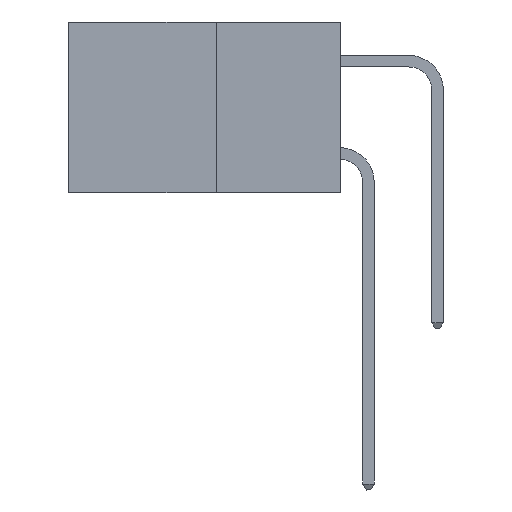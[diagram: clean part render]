
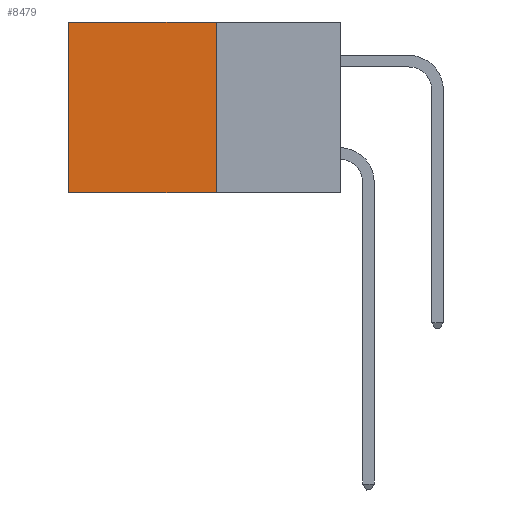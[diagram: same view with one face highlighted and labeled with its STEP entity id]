
A CAD part, left-side view. The second image highlights one B-rep face of the part: STEP entity #8479.
In plain terms, the highlighted planar face has unit normal (-1, 0, 0).
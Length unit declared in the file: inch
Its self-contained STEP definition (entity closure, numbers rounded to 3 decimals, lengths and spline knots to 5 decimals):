
#116 = VERTEX_POINT ( 'NONE', #1490 ) ;
#1490 = CARTESIAN_POINT ( 'NONE',  ( 0.277, 0.59, -0.37 ) ) ;
#2420 = VERTEX_POINT ( 'NONE', #4326 ) ;
#3546 = VERTEX_POINT ( 'NONE', #20522 ) ;
#4288 = CARTESIAN_POINT ( 'NONE',  ( 0.277, 0.27, -0.37 ) ) ;
#4326 = CARTESIAN_POINT ( 'NONE',  ( 0.277, 0.59, 0. ) ) ;
#6058 = DIRECTION ( 'NONE',  ( 0., 0., -1. ) ) ;
#6211 = DIRECTION ( 'NONE',  ( 0., 1., 0. ) ) ;
#6262 = LINE ( 'NONE', #20732, #15283 ) ;
#6589 = CARTESIAN_POINT ( 'NONE',  ( 0.277, 0.59, -0.37 ) ) ;
#8479 = ADVANCED_FACE ( 'NONE', ( #12911 ), #19672, .F. ) ;
#8651 = CARTESIAN_POINT ( 'NONE',  ( 0.277, 0.27, 0. ) ) ;
#9550 = DIRECTION ( 'NONE',  ( 1., 0., 0. ) ) ;
#10594 = DIRECTION ( 'NONE',  ( 0., 1., 0. ) ) ;
#10672 = EDGE_LOOP ( 'NONE', ( #20887, #17084, #14740, #12748 ) ) ;
#11172 = CARTESIAN_POINT ( 'NONE',  ( 0.277, 0.27, 0. ) ) ;
#11464 = LINE ( 'NONE', #4288, #19950 ) ;
#12748 = ORIENTED_EDGE ( 'NONE', *, *, #14411, .T. ) ;
#12865 = CARTESIAN_POINT ( 'NONE',  ( 0.277, 0.27, -0.37 ) ) ;
#12911 = FACE_OUTER_BOUND ( 'NONE', #10672, .T. ) ;
#13954 = VECTOR ( 'NONE', #6211, 39.37008 ) ;
#14006 = LINE ( 'NONE', #6589, #14528 ) ;
#14124 = EDGE_CURVE ( 'NONE', #3546, #116, #6262, .T. ) ;
#14411 = EDGE_CURVE ( 'NONE', #16970, #2420, #14475, .T. ) ;
#14475 = LINE ( 'NONE', #11172, #13954 ) ;
#14528 = VECTOR ( 'NONE', #18442, 39.37008 ) ;
#14740 = ORIENTED_EDGE ( 'NONE', *, *, #16077, .F. ) ;
#15283 = VECTOR ( 'NONE', #10594, 39.37008 ) ;
#16077 = EDGE_CURVE ( 'NONE', #16970, #3546, #11464, .T. ) ;
#16970 = VERTEX_POINT ( 'NONE', #8651 ) ;
#17084 = ORIENTED_EDGE ( 'NONE', *, *, #14124, .F. ) ;
#18294 = AXIS2_PLACEMENT_3D ( 'NONE', #12865, #9550, #21390 ) ;
#18442 = DIRECTION ( 'NONE',  ( 0., 0., -1. ) ) ;
#19672 = PLANE ( 'NONE',  #18294 ) ;
#19950 = VECTOR ( 'NONE', #6058, 39.37008 ) ;
#20522 = CARTESIAN_POINT ( 'NONE',  ( 0.277, 0.27, -0.37 ) ) ;
#20659 = EDGE_CURVE ( 'NONE', #2420, #116, #14006, .T. ) ;
#20732 = CARTESIAN_POINT ( 'NONE',  ( 0.277, 0.27, -0.37 ) ) ;
#20887 = ORIENTED_EDGE ( 'NONE', *, *, #20659, .T. ) ;
#21390 = DIRECTION ( 'NONE',  ( 0., 0., -1. ) ) ;
